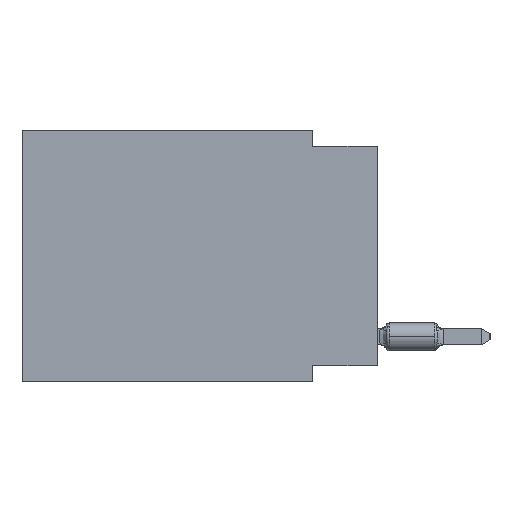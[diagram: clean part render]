
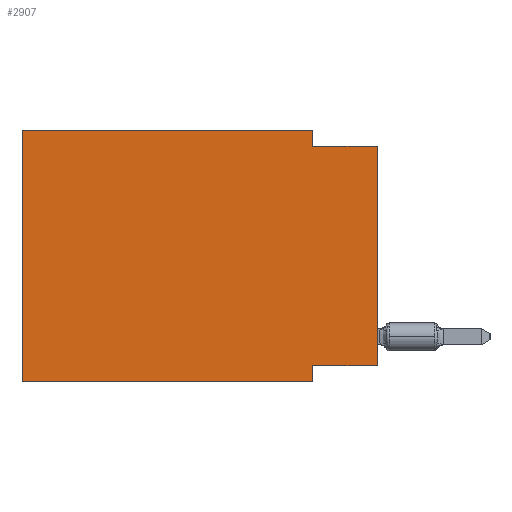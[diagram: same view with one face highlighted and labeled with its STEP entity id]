
A CAD part, left-side view. The second image highlights one B-rep face of the part: STEP entity #2907.
In plain terms, the highlighted planar face has unit normal (-1, 0, 0).
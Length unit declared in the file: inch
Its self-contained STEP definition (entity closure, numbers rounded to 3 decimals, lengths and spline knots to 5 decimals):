
#1278 = EDGE_CURVE ( 'NONE', #81500, #75532, #8788, .T. ) ;
#2907 = ADVANCED_FACE ( 'NONE', ( #21681 ), #73465, .F. ) ;
#2930 = DIRECTION ( 'NONE',  ( 0., 0., 1. ) ) ;
#3170 = EDGE_CURVE ( 'NONE', #73279, #25680, #32073, .T. ) ;
#3291 = LINE ( 'NONE', #47596, #41737 ) ;
#3562 = VECTOR ( 'NONE', #14157, 39.37008 ) ;
#3678 = DIRECTION ( 'NONE',  ( 1., 0., 0. ) ) ;
#3861 = VERTEX_POINT ( 'NONE', #16325 ) ;
#7398 = VERTEX_POINT ( 'NONE', #79572 ) ;
#8315 = LINE ( 'NONE', #59742, #3562 ) ;
#8788 = LINE ( 'NONE', #15464, #55553 ) ;
#9123 = DIRECTION ( 'NONE',  ( 0., 0., -1. ) ) ;
#9606 = CARTESIAN_POINT ( 'NONE',  ( 0., 0.55, 0. ) ) ;
#9946 = CARTESIAN_POINT ( 'NONE',  ( 0., 0.55, 0. ) ) ;
#10444 = CARTESIAN_POINT ( 'NONE',  ( 0., 0.1, -0.39 ) ) ;
#11854 = EDGE_CURVE ( 'NONE', #81500, #3861, #8315, .T. ) ;
#13124 = CARTESIAN_POINT ( 'NONE',  ( 0., 0.55, -0.39 ) ) ;
#13994 = CARTESIAN_POINT ( 'NONE',  ( 0., 0.55, 0. ) ) ;
#14157 = DIRECTION ( 'NONE',  ( 0., 1., 0. ) ) ;
#14357 = CARTESIAN_POINT ( 'NONE',  ( 0., 0.55, 0. ) ) ;
#15464 = CARTESIAN_POINT ( 'NONE',  ( 0., 0., 0. ) ) ;
#16149 = CARTESIAN_POINT ( 'NONE',  ( 0., 0.1, -0.39 ) ) ;
#16325 = CARTESIAN_POINT ( 'NONE',  ( 0., 0.1, -0.365 ) ) ;
#17134 = DIRECTION ( 'NONE',  ( 0., 0., -1. ) ) ;
#17738 = CARTESIAN_POINT ( 'NONE',  ( 0., 0.1, 0. ) ) ;
#19963 = ORIENTED_EDGE ( 'NONE', *, *, #64763, .F. ) ;
#20747 = EDGE_CURVE ( 'NONE', #7398, #73279, #61431, .T. ) ;
#21681 = FACE_OUTER_BOUND ( 'NONE', #51024, .T. ) ;
#22985 = DIRECTION ( 'NONE',  ( 0., 0., 1. ) ) ;
#23057 = ORIENTED_EDGE ( 'NONE', *, *, #64058, .T. ) ;
#25680 = VERTEX_POINT ( 'NONE', #32742 ) ;
#26038 = ORIENTED_EDGE ( 'NONE', *, *, #1278, .T. ) ;
#29333 = CARTESIAN_POINT ( 'NONE',  ( 0., 0., -0.365 ) ) ;
#31756 = VECTOR ( 'NONE', #22985, 39.37008 ) ;
#32073 = LINE ( 'NONE', #14357, #37134 ) ;
#32742 = CARTESIAN_POINT ( 'NONE',  ( 0., 0.1, 0. ) ) ;
#34743 = LINE ( 'NONE', #10444, #42286 ) ;
#36844 = VERTEX_POINT ( 'NONE', #60611 ) ;
#37134 = VECTOR ( 'NONE', #82617, 39.37008 ) ;
#41737 = VECTOR ( 'NONE', #60965, 39.37008 ) ;
#42286 = VECTOR ( 'NONE', #17134, 39.37008 ) ;
#43242 = DIRECTION ( 'NONE',  ( 0., -1., 0. ) ) ;
#43808 = AXIS2_PLACEMENT_3D ( 'NONE', #9946, #3678, #9123 ) ;
#44930 = VERTEX_POINT ( 'NONE', #16149 ) ;
#45483 = ORIENTED_EDGE ( 'NONE', *, *, #3170, .F. ) ;
#47596 = CARTESIAN_POINT ( 'NONE',  ( 0., 0., -0.025 ) ) ;
#49343 = EDGE_CURVE ( 'NONE', #36844, #75532, #3291, .T. ) ;
#50199 = CARTESIAN_POINT ( 'NONE',  ( 0., 0., -0.025 ) ) ;
#51024 = EDGE_LOOP ( 'NONE', ( #26038, #74431, #62906, #45483, #51296, #23057, #19963, #74018 ) ) ;
#51296 = ORIENTED_EDGE ( 'NONE', *, *, #20747, .F. ) ;
#55553 = VECTOR ( 'NONE', #2930, 39.37008 ) ;
#56610 = LINE ( 'NONE', #17738, #72570 ) ;
#59742 = CARTESIAN_POINT ( 'NONE',  ( 0., 0., -0.365 ) ) ;
#60611 = CARTESIAN_POINT ( 'NONE',  ( 0., 0.1, -0.025 ) ) ;
#60965 = DIRECTION ( 'NONE',  ( 0., -1., 0. ) ) ;
#61431 = LINE ( 'NONE', #9606, #31756 ) ;
#62906 = ORIENTED_EDGE ( 'NONE', *, *, #62942, .F. ) ;
#62942 = EDGE_CURVE ( 'NONE', #25680, #36844, #56610, .T. ) ;
#63295 = DIRECTION ( 'NONE',  ( 0., 0., -1. ) ) ;
#64058 = EDGE_CURVE ( 'NONE', #7398, #44930, #69973, .T. ) ;
#64763 = EDGE_CURVE ( 'NONE', #3861, #44930, #34743, .T. ) ;
#66009 = VECTOR ( 'NONE', #43242, 39.37008 ) ;
#69973 = LINE ( 'NONE', #13124, #66009 ) ;
#72570 = VECTOR ( 'NONE', #63295, 39.37008 ) ;
#73279 = VERTEX_POINT ( 'NONE', #13994 ) ;
#73465 = PLANE ( 'NONE',  #43808 ) ;
#74018 = ORIENTED_EDGE ( 'NONE', *, *, #11854, .F. ) ;
#74431 = ORIENTED_EDGE ( 'NONE', *, *, #49343, .F. ) ;
#75532 = VERTEX_POINT ( 'NONE', #50199 ) ;
#79572 = CARTESIAN_POINT ( 'NONE',  ( 0., 0.55, -0.39 ) ) ;
#81500 = VERTEX_POINT ( 'NONE', #29333 ) ;
#82617 = DIRECTION ( 'NONE',  ( 0., -1., 0. ) ) ;
